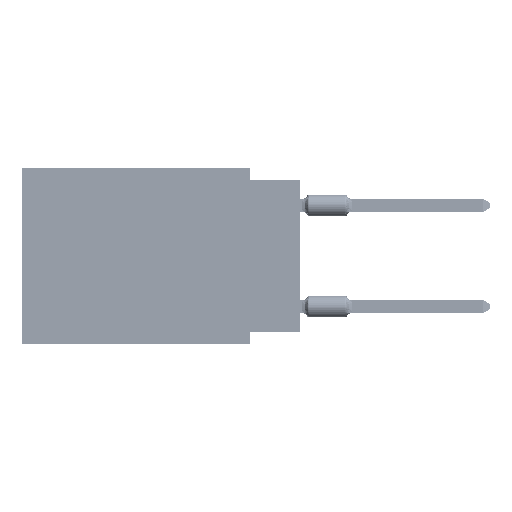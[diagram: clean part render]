
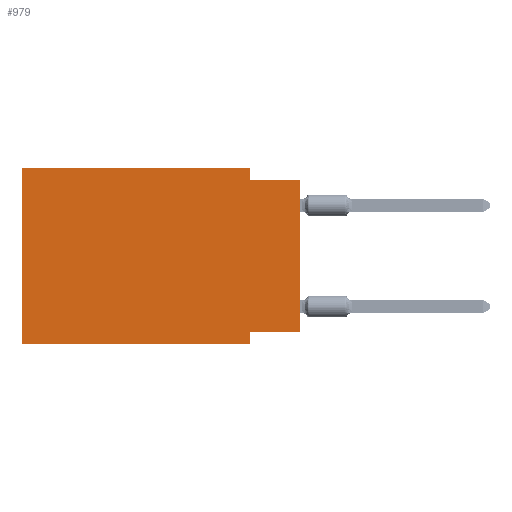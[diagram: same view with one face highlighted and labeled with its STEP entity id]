
A CAD part, left-side view. The second image highlights one B-rep face of the part: STEP entity #979.
In plain terms, the highlighted planar face has unit normal (-1, 0, 0).
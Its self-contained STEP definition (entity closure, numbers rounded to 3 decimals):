
#283 = DIRECTION ( 'NONE',  ( 0., -1., 0. ) ) ;
#979 = ADVANCED_FACE ( 'NONE', ( #24697 ), #94066, .F. ) ;
#4192 = VECTOR ( 'NONE', #283, 1000. ) ;
#7078 = ORIENTED_EDGE ( 'NONE', *, *, #46485, .F. ) ;
#8232 = LINE ( 'NONE', #26966, #55301 ) ;
#8633 = CARTESIAN_POINT ( 'NONE',  ( 0., 2.54, -8.255 ) ) ;
#9381 = LINE ( 'NONE', #18466, #4192 ) ;
#9923 = DIRECTION ( 'NONE',  ( 0., -1., 0. ) ) ;
#10268 = ORIENTED_EDGE ( 'NONE', *, *, #76172, .F. ) ;
#12278 = CARTESIAN_POINT ( 'NONE',  ( 0., 2.54, 0. ) ) ;
#16522 = VERTEX_POINT ( 'NONE', #8633 ) ;
#18466 = CARTESIAN_POINT ( 'NONE',  ( 0., 0., -0.635 ) ) ;
#18555 = VECTOR ( 'NONE', #109122, 1000. ) ;
#19036 = EDGE_CURVE ( 'NONE', #100716, #32899, #8232, .T. ) ;
#19323 = LINE ( 'NONE', #48836, #18555 ) ;
#22506 = VERTEX_POINT ( 'NONE', #12278 ) ;
#22943 = ORIENTED_EDGE ( 'NONE', *, *, #81749, .F. ) ;
#24697 = FACE_OUTER_BOUND ( 'NONE', #90106, .T. ) ;
#26560 = VERTEX_POINT ( 'NONE', #40537 ) ;
#26966 = CARTESIAN_POINT ( 'NONE',  ( 0., 13.97, -8.89 ) ) ;
#32899 = VERTEX_POINT ( 'NONE', #42032 ) ;
#38166 = EDGE_CURVE ( 'NONE', #22506, #26560, #97010, .T. ) ;
#38521 = VECTOR ( 'NONE', #111735, 1000. ) ;
#40537 = CARTESIAN_POINT ( 'NONE',  ( 0., 2.54, -0.635 ) ) ;
#41698 = CARTESIAN_POINT ( 'NONE',  ( 0., 13.97, 0. ) ) ;
#42032 = CARTESIAN_POINT ( 'NONE',  ( 0., 2.54, -8.89 ) ) ;
#42318 = DIRECTION ( 'NONE',  ( 1., 0., 0. ) ) ;
#45794 = CARTESIAN_POINT ( 'NONE',  ( 0., 2.54, 0. ) ) ;
#46485 = EDGE_CURVE ( 'NONE', #83881, #22506, #91967, .T. ) ;
#48188 = CARTESIAN_POINT ( 'NONE',  ( 0., 13.97, 0. ) ) ;
#48836 = CARTESIAN_POINT ( 'NONE',  ( 0., 0., -8.255 ) ) ;
#53478 = VERTEX_POINT ( 'NONE', #61852 ) ;
#54785 = VECTOR ( 'NONE', #97564, 1000. ) ;
#55301 = VECTOR ( 'NONE', #9923, 1000. ) ;
#55852 = VECTOR ( 'NONE', #82888, 1000. ) ;
#56087 = ORIENTED_EDGE ( 'NONE', *, *, #108121, .F. ) ;
#56994 = CARTESIAN_POINT ( 'NONE',  ( 0., 2.54, -8.89 ) ) ;
#58278 = LINE ( 'NONE', #83892, #38521 ) ;
#61852 = CARTESIAN_POINT ( 'NONE',  ( 0., 0., -0.635 ) ) ;
#63544 = CARTESIAN_POINT ( 'NONE',  ( 0., 13.97, 0. ) ) ;
#65557 = ORIENTED_EDGE ( 'NONE', *, *, #38166, .F. ) ;
#69044 = VECTOR ( 'NONE', #89988, 1000. ) ;
#75207 = EDGE_CURVE ( 'NONE', #85538, #16522, #19323, .T. ) ;
#76172 = EDGE_CURVE ( 'NONE', #100716, #83881, #83824, .T. ) ;
#77592 = CARTESIAN_POINT ( 'NONE',  ( 0., 13.97, 0. ) ) ;
#81749 = EDGE_CURVE ( 'NONE', #26560, #53478, #9381, .T. ) ;
#82247 = ORIENTED_EDGE ( 'NONE', *, *, #19036, .T. ) ;
#82322 = VECTOR ( 'NONE', #111087, 1000. ) ;
#82888 = DIRECTION ( 'NONE',  ( 0., -1., 0. ) ) ;
#83361 = ORIENTED_EDGE ( 'NONE', *, *, #75207, .F. ) ;
#83824 = LINE ( 'NONE', #41698, #82322 ) ;
#83881 = VERTEX_POINT ( 'NONE', #63544 ) ;
#83892 = CARTESIAN_POINT ( 'NONE',  ( 0., 0., 0. ) ) ;
#85534 = DIRECTION ( 'NONE',  ( 0., 0., -1. ) ) ;
#85538 = VERTEX_POINT ( 'NONE', #89599 ) ;
#89599 = CARTESIAN_POINT ( 'NONE',  ( 0., 0., -8.255 ) ) ;
#89988 = DIRECTION ( 'NONE',  ( 0., 0., -1. ) ) ;
#90106 = EDGE_LOOP ( 'NONE', ( #94200, #22943, #65557, #7078, #10268, #82247, #56087, #83361 ) ) ;
#90368 = CARTESIAN_POINT ( 'NONE',  ( 0., 13.97, -8.89 ) ) ;
#91967 = LINE ( 'NONE', #48188, #55852 ) ;
#94066 = PLANE ( 'NONE',  #94761 ) ;
#94200 = ORIENTED_EDGE ( 'NONE', *, *, #110337, .T. ) ;
#94761 = AXIS2_PLACEMENT_3D ( 'NONE', #77592, #42318, #85534 ) ;
#97010 = LINE ( 'NONE', #45794, #54785 ) ;
#97564 = DIRECTION ( 'NONE',  ( 0., 0., -1. ) ) ;
#100716 = VERTEX_POINT ( 'NONE', #90368 ) ;
#100783 = LINE ( 'NONE', #56994, #69044 ) ;
#108121 = EDGE_CURVE ( 'NONE', #16522, #32899, #100783, .T. ) ;
#109122 = DIRECTION ( 'NONE',  ( 0., 1., 0. ) ) ;
#110337 = EDGE_CURVE ( 'NONE', #85538, #53478, #58278, .T. ) ;
#111087 = DIRECTION ( 'NONE',  ( 0., 0., 1. ) ) ;
#111735 = DIRECTION ( 'NONE',  ( 0., 0., 1. ) ) ;
